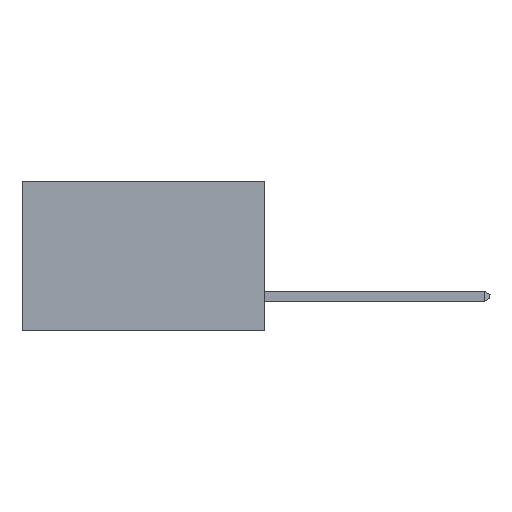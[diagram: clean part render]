
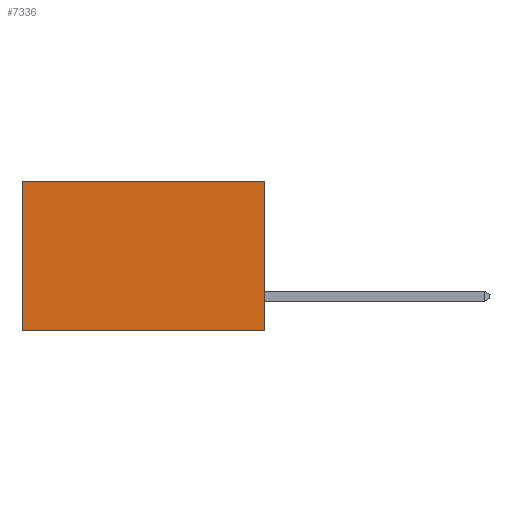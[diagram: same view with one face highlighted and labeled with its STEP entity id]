
A CAD part, left-side view. The second image highlights one B-rep face of the part: STEP entity #7336.
In plain terms, the highlighted planar face has unit normal (-1, 0, 0).
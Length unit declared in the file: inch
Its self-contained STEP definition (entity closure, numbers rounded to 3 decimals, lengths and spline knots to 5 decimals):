
#330 = LINE ( 'NONE', #11884, #4122 ) ;
#557 = VECTOR ( 'NONE', #12833, 39.37008 ) ;
#1056 = EDGE_CURVE ( 'NONE', #5641, #14042, #3149, .T. ) ;
#1828 = EDGE_CURVE ( 'NONE', #14042, #9364, #3305, .T. ) ;
#2405 = LINE ( 'NONE', #14027, #557 ) ;
#3149 = LINE ( 'NONE', #6528, #9834 ) ;
#3305 = LINE ( 'NONE', #11481, #9925 ) ;
#4122 = VECTOR ( 'NONE', #8202, 39.37008 ) ;
#5095 = ORIENTED_EDGE ( 'NONE', *, *, #1828, .F. ) ;
#5367 = CARTESIAN_POINT ( 'NONE',  ( 0.2615, 0., 0. ) ) ;
#5641 = VERTEX_POINT ( 'NONE', #5367 ) ;
#6005 = CARTESIAN_POINT ( 'NONE',  ( 0.2615, 0.6, 0. ) ) ;
#6528 = CARTESIAN_POINT ( 'NONE',  ( 0.2615, 0., -0.37 ) ) ;
#6904 = DIRECTION ( 'NONE',  ( 0., 1., 0. ) ) ;
#7287 = VERTEX_POINT ( 'NONE', #6005 ) ;
#7336 = ADVANCED_FACE ( 'NONE', ( #8562 ), #8627, .F. ) ;
#7633 = ORIENTED_EDGE ( 'NONE', *, *, #1056, .F. ) ;
#8202 = DIRECTION ( 'NONE',  ( 0., 0., -1. ) ) ;
#8562 = FACE_OUTER_BOUND ( 'NONE', #9422, .T. ) ;
#8627 = PLANE ( 'NONE',  #14697 ) ;
#8799 = EDGE_CURVE ( 'NONE', #5641, #7287, #2405, .T. ) ;
#8851 = DIRECTION ( 'NONE',  ( 0., 0., -1. ) ) ;
#9364 = VERTEX_POINT ( 'NONE', #11396 ) ;
#9422 = EDGE_LOOP ( 'NONE', ( #14765, #5095, #7633, #11425 ) ) ;
#9834 = VECTOR ( 'NONE', #8851, 39.37008 ) ;
#9925 = VECTOR ( 'NONE', #6904, 39.37008 ) ;
#11396 = CARTESIAN_POINT ( 'NONE',  ( 0.2615, 0.6, -0.37 ) ) ;
#11425 = ORIENTED_EDGE ( 'NONE', *, *, #8799, .T. ) ;
#11481 = CARTESIAN_POINT ( 'NONE',  ( 0.2615, 0., -0.37 ) ) ;
#11613 = EDGE_CURVE ( 'NONE', #7287, #9364, #330, .T. ) ;
#11884 = CARTESIAN_POINT ( 'NONE',  ( 0.2615, 0.6, -0.37 ) ) ;
#12833 = DIRECTION ( 'NONE',  ( 0., 1., 0. ) ) ;
#12868 = CARTESIAN_POINT ( 'NONE',  ( 0.2615, 0., -0.37 ) ) ;
#13073 = DIRECTION ( 'NONE',  ( 1., 0., 0. ) ) ;
#13139 = DIRECTION ( 'NONE',  ( 0., 0., -1. ) ) ;
#14027 = CARTESIAN_POINT ( 'NONE',  ( 0.2615, 0., 0. ) ) ;
#14042 = VERTEX_POINT ( 'NONE', #12868 ) ;
#14336 = CARTESIAN_POINT ( 'NONE',  ( 0.2615, 0., -0.37 ) ) ;
#14697 = AXIS2_PLACEMENT_3D ( 'NONE', #14336, #13073, #13139 ) ;
#14765 = ORIENTED_EDGE ( 'NONE', *, *, #11613, .T. ) ;
